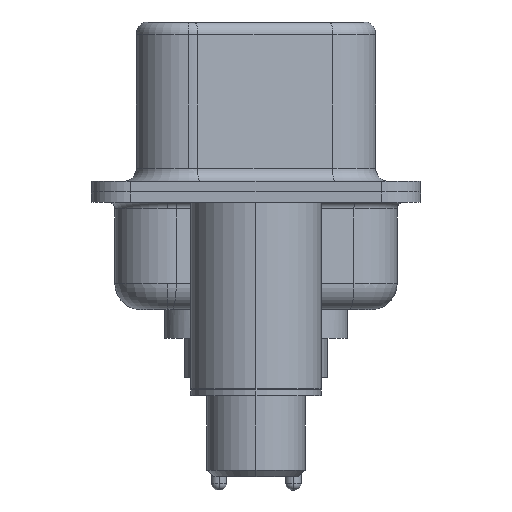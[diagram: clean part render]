
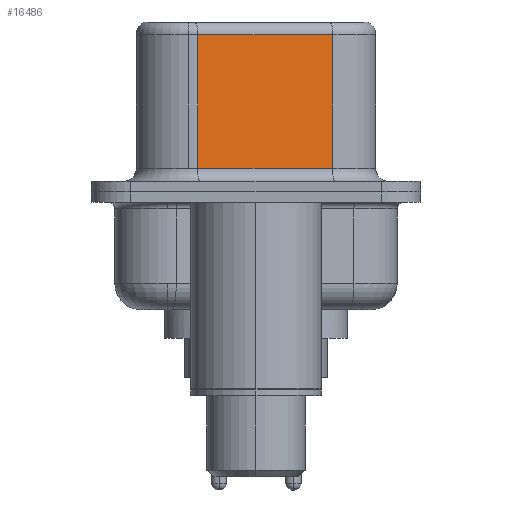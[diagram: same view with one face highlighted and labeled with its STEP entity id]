
A CAD part, left-side view. The second image highlights one B-rep face of the part: STEP entity #16486.
In plain terms, the highlighted planar face has unit normal (-0.985, -0.174, 0).
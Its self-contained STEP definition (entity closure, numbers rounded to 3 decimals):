
#55 = VECTOR ( 'NONE', #1124, 1000. ) ;
#612 = VERTEX_POINT ( 'NONE', #9684 ) ;
#864 = AXIS2_PLACEMENT_3D ( 'NONE', #1767, #11940, #3249 ) ;
#956 = ORIENTED_EDGE ( 'NONE', *, *, #3957, .T. ) ;
#1124 = DIRECTION ( 'NONE',  ( -0.174, 0.985, 0. ) ) ;
#1767 = CARTESIAN_POINT ( 'NONE',  ( 4.585, -2.927, 6.52 ) ) ;
#2561 = EDGE_LOOP ( 'NONE', ( #10286, #16785, #956, #15504 ) ) ;
#2970 = EDGE_CURVE ( 'NONE', #612, #15268, #8135, .T. ) ;
#3249 = DIRECTION ( 'NONE',  ( -0.174, 0.985, 0. ) ) ;
#3957 = EDGE_CURVE ( 'NONE', #9976, #18870, #16847, .T. ) ;
#4289 = VECTOR ( 'NONE', #18817, 1000. ) ;
#8031 = EDGE_CURVE ( 'NONE', #612, #9976, #18575, .T. ) ;
#8135 = LINE ( 'NONE', #18701, #4289 ) ;
#8366 = CARTESIAN_POINT ( 'NONE',  ( 4.585, -2.927, 6.02 ) ) ;
#9014 = VECTOR ( 'NONE', #18340, 1000. ) ;
#9460 = VECTOR ( 'NONE', #14322, 1000. ) ;
#9527 = CARTESIAN_POINT ( 'NONE',  ( 4.585, -2.927, 0.9 ) ) ;
#9684 = CARTESIAN_POINT ( 'NONE',  ( 4.585, -2.927, 6.02 ) ) ;
#9976 = VERTEX_POINT ( 'NONE', #18545 ) ;
#10030 = CARTESIAN_POINT ( 'NONE',  ( 4.585, -2.927, 0.9 ) ) ;
#10286 = ORIENTED_EDGE ( 'NONE', *, *, #2970, .F. ) ;
#11870 = PLANE ( 'NONE',  #864 ) ;
#11940 = DIRECTION ( 'NONE',  ( 0.985, 0.174, 0. ) ) ;
#12725 = EDGE_CURVE ( 'NONE', #18870, #15268, #12914, .T. ) ;
#12914 = LINE ( 'NONE', #9527, #9014 ) ;
#13039 = CARTESIAN_POINT ( 'NONE',  ( 3.675, 2.233, 0.9 ) ) ;
#13849 = CARTESIAN_POINT ( 'NONE',  ( 3.675, 2.233, 6.52 ) ) ;
#14322 = DIRECTION ( 'NONE',  ( 0., 0., -1. ) ) ;
#15268 = VERTEX_POINT ( 'NONE', #10030 ) ;
#15504 = ORIENTED_EDGE ( 'NONE', *, *, #12725, .T. ) ;
#16486 = ADVANCED_FACE ( 'NONE', ( #16662 ), #11870, .F. ) ;
#16662 = FACE_OUTER_BOUND ( 'NONE', #2561, .T. ) ;
#16785 = ORIENTED_EDGE ( 'NONE', *, *, #8031, .T. ) ;
#16847 = LINE ( 'NONE', #13849, #9460 ) ;
#18340 = DIRECTION ( 'NONE',  ( 0.174, -0.985, 0. ) ) ;
#18545 = CARTESIAN_POINT ( 'NONE',  ( 3.675, 2.233, 6.02 ) ) ;
#18575 = LINE ( 'NONE', #8366, #55 ) ;
#18701 = CARTESIAN_POINT ( 'NONE',  ( 4.585, -2.927, 6.52 ) ) ;
#18817 = DIRECTION ( 'NONE',  ( 0., 0., -1. ) ) ;
#18870 = VERTEX_POINT ( 'NONE', #13039 ) ;
